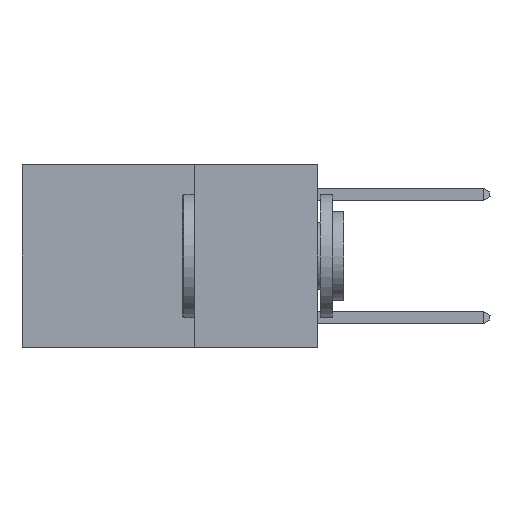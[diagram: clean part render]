
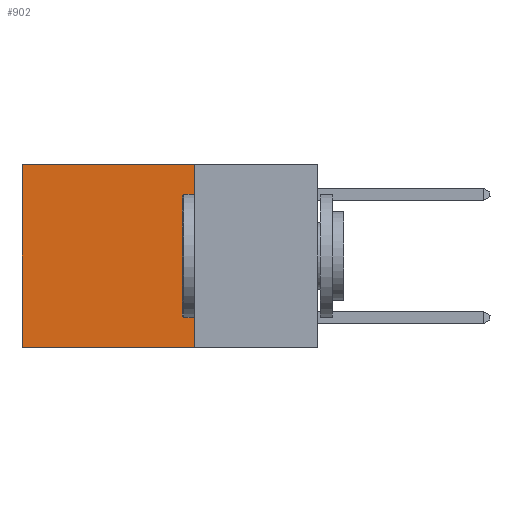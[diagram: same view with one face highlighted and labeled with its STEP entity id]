
A CAD part, left-side view. The second image highlights one B-rep face of the part: STEP entity #902.
In plain terms, the highlighted planar face has unit normal (-1, 0, 0).
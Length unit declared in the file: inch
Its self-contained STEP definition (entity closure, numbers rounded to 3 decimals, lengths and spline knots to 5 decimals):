
#576 = EDGE_CURVE ( 'NONE', #8548, #1254, #15319, .T. ) ;
#902 = ADVANCED_FACE ( 'NONE', ( #5856 ), #12927, .F. ) ;
#1254 = VERTEX_POINT ( 'NONE', #23651 ) ;
#1641 = DIRECTION ( 'NONE',  ( 0., 0., -1. ) ) ;
#1758 = CARTESIAN_POINT ( 'NONE',  ( 0.2625, 0.25, 0. ) ) ;
#1875 = EDGE_LOOP ( 'NONE', ( #15741, #19164, #24405, #24272 ) ) ;
#2443 = LINE ( 'NONE', #8886, #27748 ) ;
#3633 = VECTOR ( 'NONE', #28700, 39.37008 ) ;
#3672 = DIRECTION ( 'NONE',  ( 1., 0., 0. ) ) ;
#4304 = VECTOR ( 'NONE', #19148, 39.37008 ) ;
#5856 = FACE_OUTER_BOUND ( 'NONE', #1875, .T. ) ;
#8548 = VERTEX_POINT ( 'NONE', #12498 ) ;
#8667 = VERTEX_POINT ( 'NONE', #9087 ) ;
#8789 = CARTESIAN_POINT ( 'NONE',  ( 0.2625, 0.6, 0. ) ) ;
#8886 = CARTESIAN_POINT ( 'NONE',  ( 0.2625, 0.25, -0.37 ) ) ;
#9087 = CARTESIAN_POINT ( 'NONE',  ( 0.2625, 0.6, -0.37 ) ) ;
#9443 = EDGE_CURVE ( 'NONE', #1254, #8667, #2443, .T. ) ;
#10863 = CARTESIAN_POINT ( 'NONE',  ( 0.2625, 0.6, 0. ) ) ;
#12101 = AXIS2_PLACEMENT_3D ( 'NONE', #1758, #3672, #12495 ) ;
#12495 = DIRECTION ( 'NONE',  ( 0., 0., -1. ) ) ;
#12498 = CARTESIAN_POINT ( 'NONE',  ( 0.2625, 0.25, 0. ) ) ;
#12927 = PLANE ( 'NONE',  #12101 ) ;
#15100 = EDGE_CURVE ( 'NONE', #17081, #8667, #17064, .T. ) ;
#15319 = LINE ( 'NONE', #19717, #3633 ) ;
#15376 = DIRECTION ( 'NONE',  ( 0., 1., 0. ) ) ;
#15741 = ORIENTED_EDGE ( 'NONE', *, *, #15100, .T. ) ;
#17064 = LINE ( 'NONE', #10863, #26304 ) ;
#17081 = VERTEX_POINT ( 'NONE', #8789 ) ;
#19148 = DIRECTION ( 'NONE',  ( 0., 1., 0. ) ) ;
#19164 = ORIENTED_EDGE ( 'NONE', *, *, #9443, .F. ) ;
#19717 = CARTESIAN_POINT ( 'NONE',  ( 0.2625, 0.25, 0. ) ) ;
#20920 = CARTESIAN_POINT ( 'NONE',  ( 0.2625, 0.25, 0. ) ) ;
#23651 = CARTESIAN_POINT ( 'NONE',  ( 0.2625, 0.25, -0.37 ) ) ;
#24272 = ORIENTED_EDGE ( 'NONE', *, *, #27007, .T. ) ;
#24405 = ORIENTED_EDGE ( 'NONE', *, *, #576, .F. ) ;
#25184 = LINE ( 'NONE', #20920, #4304 ) ;
#26304 = VECTOR ( 'NONE', #1641, 39.37008 ) ;
#27007 = EDGE_CURVE ( 'NONE', #8548, #17081, #25184, .T. ) ;
#27748 = VECTOR ( 'NONE', #15376, 39.37008 ) ;
#28700 = DIRECTION ( 'NONE',  ( 0., 0., -1. ) ) ;
